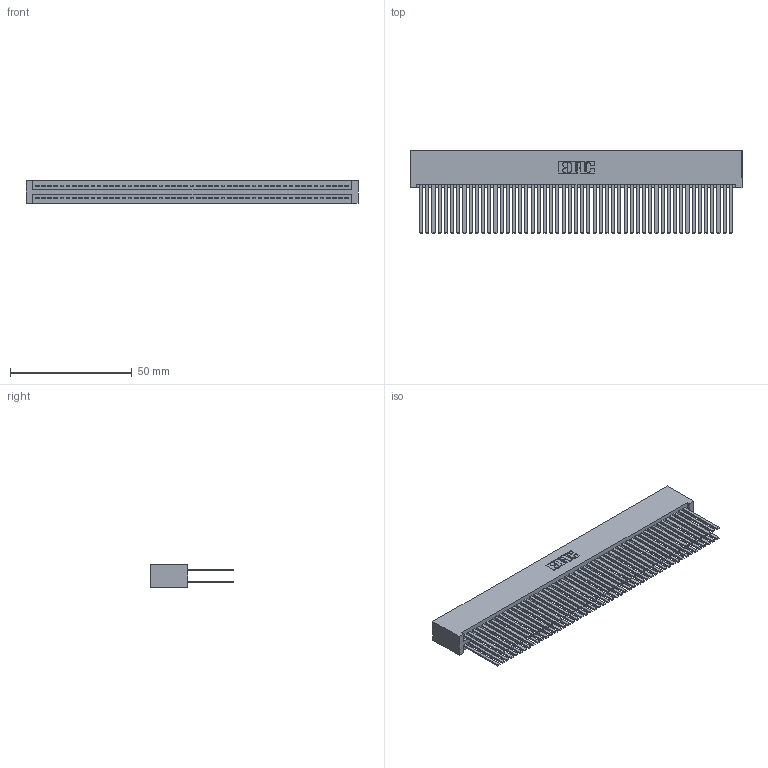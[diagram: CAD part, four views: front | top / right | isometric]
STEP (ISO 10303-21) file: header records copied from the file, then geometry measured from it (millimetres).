
FILE_DESCRIPTION (( 'STEP AP203' ), '1' );
FILE_NAME ('395-102-544-201.STEP', '2018-11-30T08:07:11', ( '' ), ( '' ), 'SwSTEP 2.0', 'SolidWorks 2016', '' );
FILE_SCHEMA (( 'CONFIG_CONTROL_DESIGN' ));
Length unit declared in the file: inch
Products named in the file (3): 345-292-001_345-293-144; 395-102-544-201; 345 Part_No Mounting Lugs
Assembly tree (103 placements, depth 2):
  395-102-544-201
    345 Part_No Mounting Lugs
    345-292-001_345-293-144  x102
Bounding box: 136.14 x 33.96 x 9.4 mm (x, y, z)
Volume: 15354.5 mm3; surface area: 27364.8 mm2
Topology: 103 solids, 103 shells, 4606 faces, 13679 edges, 8982 vertices
Faces by surface type: plane 3034, cylinder 1572
Entity records: 38343 total; most frequent: CARTESIAN_POINT 6416, ORIENTED_EDGE 6350, DIRECTION 5639, EDGE_CURVE 3175, VECTOR 2851, LINE 2851, VERTEX_POINT 2114, AXIS2_PLACEMENT_3D 1394
